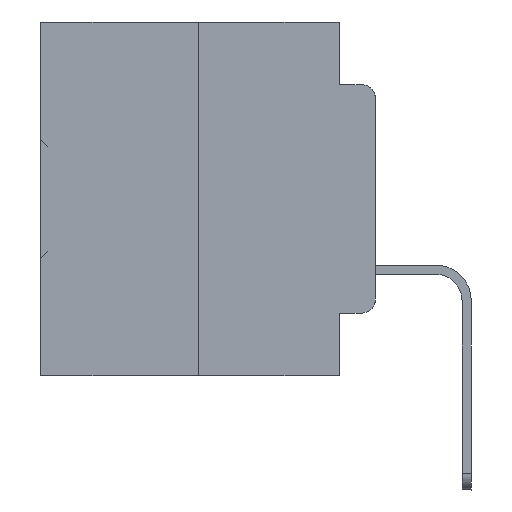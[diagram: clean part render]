
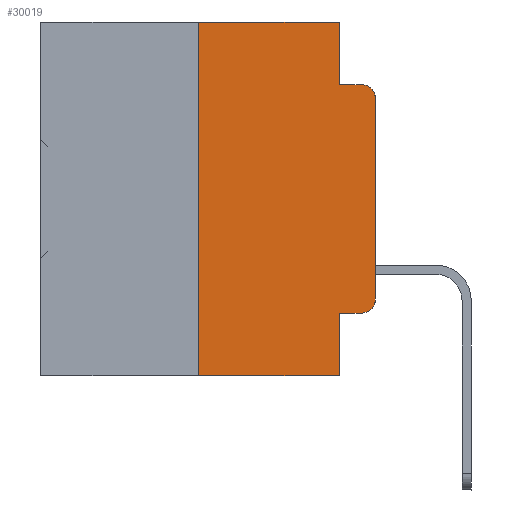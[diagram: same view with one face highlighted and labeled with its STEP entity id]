
A CAD part, left-side view. The second image highlights one B-rep face of the part: STEP entity #30019.
In plain terms, the highlighted planar face has unit normal (-1, 0, 0).
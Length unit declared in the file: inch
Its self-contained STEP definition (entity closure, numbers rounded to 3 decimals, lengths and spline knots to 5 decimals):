
#333 = CARTESIAN_POINT ( 'NONE',  ( 0., 0.25, 0. ) ) ;
#648 = ORIENTED_EDGE ( 'NONE', *, *, #37923, .F. ) ;
#762 = DIRECTION ( 'NONE',  ( -1., 0., 0. ) ) ;
#2080 = DIRECTION ( 'NONE',  ( -1., 0., 0. ) ) ;
#2221 = LINE ( 'NONE', #20811, #9169 ) ;
#2233 = AXIS2_PLACEMENT_3D ( 'NONE', #27800, #27927, #24837 ) ;
#2409 = VECTOR ( 'NONE', #19041, 39.37008 ) ;
#2430 = CARTESIAN_POINT ( 'NONE',  ( 0., 0.051, 0. ) ) ;
#4011 = EDGE_LOOP ( 'NONE', ( #26955, #19394, #27221, #648, #16730, #31621, #23712, #20468, #21249, #14084 ) ) ;
#5156 = LINE ( 'NONE', #16941, #30854 ) ;
#5209 = FACE_OUTER_BOUND ( 'NONE', #4011, .T. ) ;
#5228 = CIRCLE ( 'NONE', #19438, 0.02 ) ;
#6002 = EDGE_CURVE ( 'NONE', #14359, #10385, #22403, .T. ) ;
#6123 = DIRECTION ( 'NONE',  ( 0., 0., 1. ) ) ;
#6715 = DIRECTION ( 'NONE',  ( 0., -1., 0. ) ) ;
#6729 = CARTESIAN_POINT ( 'NONE',  ( 0., 0.051, -0.0885 ) ) ;
#7262 = PLANE ( 'NONE',  #2233 ) ;
#7419 = CARTESIAN_POINT ( 'NONE',  ( 0., 0., -0.3915 ) ) ;
#7617 = CARTESIAN_POINT ( 'NONE',  ( 0., 0.02, -0.3915 ) ) ;
#8071 = DIRECTION ( 'NONE',  ( 0., 0., -1. ) ) ;
#8288 = CARTESIAN_POINT ( 'NONE',  ( 0., 0., 0. ) ) ;
#8532 = DIRECTION ( 'NONE',  ( 0., 0., 1. ) ) ;
#8777 = EDGE_CURVE ( 'NONE', #17568, #24395, #25010, .T. ) ;
#9082 = CARTESIAN_POINT ( 'NONE',  ( 0., 0.02, -0.4115 ) ) ;
#9146 = EDGE_CURVE ( 'NONE', #10385, #37085, #5228, .T. ) ;
#9169 = VECTOR ( 'NONE', #21059, 39.37008 ) ;
#10337 = LINE ( 'NONE', #333, #11240 ) ;
#10385 = VERTEX_POINT ( 'NONE', #9082 ) ;
#11240 = VECTOR ( 'NONE', #6123, 39.37008 ) ;
#11766 = CARTESIAN_POINT ( 'NONE',  ( 0., 0.051, -0.4115 ) ) ;
#11967 = EDGE_CURVE ( 'NONE', #37610, #24395, #34123, .T. ) ;
#13271 = DIRECTION ( 'NONE',  ( 0., 0., -1. ) ) ;
#14084 = ORIENTED_EDGE ( 'NONE', *, *, #9146, .T. ) ;
#14359 = VERTEX_POINT ( 'NONE', #11766 ) ;
#14532 = CARTESIAN_POINT ( 'NONE',  ( 0., 0.051, -0.5 ) ) ;
#14589 = VECTOR ( 'NONE', #6715, 39.37008 ) ;
#15732 = CARTESIAN_POINT ( 'NONE',  ( 0., 0.02, -0.1085 ) ) ;
#15833 = CARTESIAN_POINT ( 'NONE',  ( 0., 0.051, -0.0885 ) ) ;
#16082 = CARTESIAN_POINT ( 'NONE',  ( 0., 0., -0.1085 ) ) ;
#16730 = ORIENTED_EDGE ( 'NONE', *, *, #19814, .F. ) ;
#16904 = CARTESIAN_POINT ( 'NONE',  ( 0., 0.473, 0. ) ) ;
#16941 = CARTESIAN_POINT ( 'NONE',  ( 0., 0.051, 0. ) ) ;
#17128 = EDGE_CURVE ( 'NONE', #14359, #32470, #17697, .T. ) ;
#17568 = VERTEX_POINT ( 'NONE', #16082 ) ;
#17697 = LINE ( 'NONE', #25921, #28766 ) ;
#18246 = EDGE_CURVE ( 'NONE', #21622, #26515, #10337, .T. ) ;
#19041 = DIRECTION ( 'NONE',  ( 0., -1., 0. ) ) ;
#19320 = EDGE_CURVE ( 'NONE', #21622, #32470, #2221, .T. ) ;
#19394 = ORIENTED_EDGE ( 'NONE', *, *, #8777, .T. ) ;
#19438 = AXIS2_PLACEMENT_3D ( 'NONE', #7617, #2080, #13271 ) ;
#19603 = DIRECTION ( 'NONE',  ( 0., -1., 0. ) ) ;
#19814 = EDGE_CURVE ( 'NONE', #26515, #22609, #37049, .T. ) ;
#20468 = ORIENTED_EDGE ( 'NONE', *, *, #17128, .F. ) ;
#20811 = CARTESIAN_POINT ( 'NONE',  ( 0., 0.473, -0.5 ) ) ;
#21001 = EDGE_CURVE ( 'NONE', #37085, #17568, #32381, .T. ) ;
#21059 = DIRECTION ( 'NONE',  ( 0., -1., 0. ) ) ;
#21249 = ORIENTED_EDGE ( 'NONE', *, *, #6002, .T. ) ;
#21622 = VERTEX_POINT ( 'NONE', #32209 ) ;
#22275 = CARTESIAN_POINT ( 'NONE',  ( 0., 0.25, 0. ) ) ;
#22403 = LINE ( 'NONE', #23924, #14589 ) ;
#22609 = VERTEX_POINT ( 'NONE', #2430 ) ;
#22839 = CARTESIAN_POINT ( 'NONE',  ( 0., 0.02, -0.0885 ) ) ;
#23712 = ORIENTED_EDGE ( 'NONE', *, *, #19320, .T. ) ;
#23924 = CARTESIAN_POINT ( 'NONE',  ( 0., 0.051, -0.4115 ) ) ;
#24395 = VERTEX_POINT ( 'NONE', #22839 ) ;
#24837 = DIRECTION ( 'NONE',  ( 0., 0., -1. ) ) ;
#25010 = CIRCLE ( 'NONE', #31706, 0.02 ) ;
#25921 = CARTESIAN_POINT ( 'NONE',  ( 0., 0.051, 0. ) ) ;
#25975 = DIRECTION ( 'NONE',  ( 0., 0., -1. ) ) ;
#26515 = VERTEX_POINT ( 'NONE', #22275 ) ;
#26955 = ORIENTED_EDGE ( 'NONE', *, *, #21001, .T. ) ;
#27221 = ORIENTED_EDGE ( 'NONE', *, *, #11967, .F. ) ;
#27800 = CARTESIAN_POINT ( 'NONE',  ( 0., 0.473, 0. ) ) ;
#27927 = DIRECTION ( 'NONE',  ( 1., 0., 0. ) ) ;
#28766 = VECTOR ( 'NONE', #8071, 39.37008 ) ;
#30017 = DIRECTION ( 'NONE',  ( 0., 0., -1. ) ) ;
#30019 = ADVANCED_FACE ( 'NONE', ( #5209 ), #7262, .F. ) ;
#30064 = VECTOR ( 'NONE', #8532, 39.37008 ) ;
#30854 = VECTOR ( 'NONE', #25975, 39.37008 ) ;
#31621 = ORIENTED_EDGE ( 'NONE', *, *, #18246, .F. ) ;
#31706 = AXIS2_PLACEMENT_3D ( 'NONE', #15732, #762, #30017 ) ;
#32209 = CARTESIAN_POINT ( 'NONE',  ( 0., 0.25, -0.5 ) ) ;
#32381 = LINE ( 'NONE', #8288, #30064 ) ;
#32456 = VECTOR ( 'NONE', #19603, 39.37008 ) ;
#32470 = VERTEX_POINT ( 'NONE', #14532 ) ;
#34123 = LINE ( 'NONE', #15833, #2409 ) ;
#37049 = LINE ( 'NONE', #16904, #32456 ) ;
#37085 = VERTEX_POINT ( 'NONE', #7419 ) ;
#37610 = VERTEX_POINT ( 'NONE', #6729 ) ;
#37923 = EDGE_CURVE ( 'NONE', #22609, #37610, #5156, .T. ) ;
